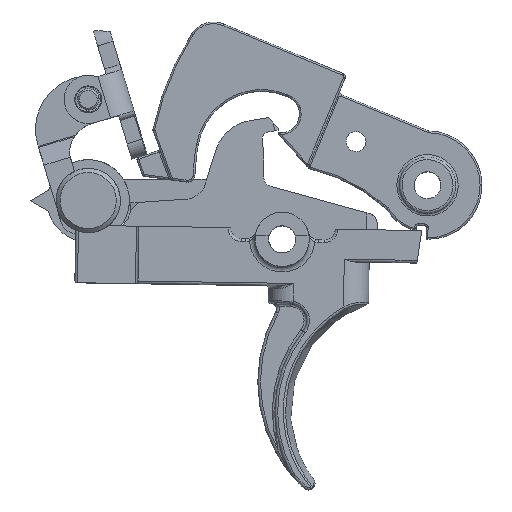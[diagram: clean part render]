
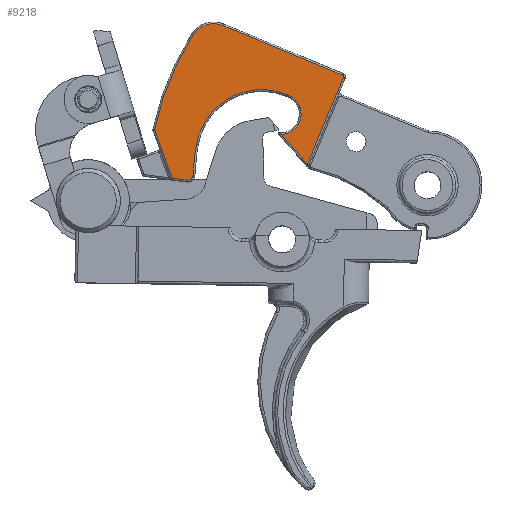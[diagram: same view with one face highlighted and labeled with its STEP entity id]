
A CAD part, top view. The second image highlights one B-rep face of the part: STEP entity #9218.
In plain terms, the highlighted planar face has unit normal (0, 0, 1).
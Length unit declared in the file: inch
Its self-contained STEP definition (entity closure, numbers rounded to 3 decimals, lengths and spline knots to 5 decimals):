
#1012=CIRCLE('',#10325,0.01);
#1057=CIRCLE('',#10414,0.031);
#1059=CIRCLE('',#10417,1.36056);
#1061=CIRCLE('',#10420,0.385);
#1063=CIRCLE('',#10424,0.11935);
#1076=CIRCLE('',#10447,0.141);
#1078=CIRCLE('',#10450,1.615);
#1248=PLANE('',#10457);
#1818=FACE_OUTER_BOUND('',#2459,.T.);
#2459=EDGE_LOOP('',(#8425,#8426,#8427,#8428,#8429,#8430,#8431,#8432,#8433,
#8434,#8435,#8436,#8437));
#2919=LINE('',#24606,#3483);
#2961=LINE('',#24880,#3525);
#3017=LINE('',#25762,#3581);
#3021=LINE('',#25791,#3585);
#3023=LINE('',#25796,#3587);
#3024=LINE('',#25798,#3588);
#3483=VECTOR('',#12593,0.3937);
#3525=VECTOR('',#12785,0.3937);
#3581=VECTOR('',#13173,0.3937);
#3585=VECTOR('',#13215,0.3937);
#3587=VECTOR('',#13221,0.3937);
#3588=VECTOR('',#13224,0.3937);
#4276=VERTEX_POINT('',#24519);
#4290=VERTEX_POINT('',#24604);
#4350=VERTEX_POINT('',#24866);
#4353=VERTEX_POINT('',#24878);
#4406=VERTEX_POINT('',#25387);
#4438=VERTEX_POINT('',#25682);
#4440=VERTEX_POINT('',#25748);
#4441=VERTEX_POINT('',#25752);
#4442=VERTEX_POINT('',#25756);
#4443=VERTEX_POINT('',#25760);
#4448=VERTEX_POINT('',#25782);
#4450=VERTEX_POINT('',#25794);
#4452=VERTEX_POINT('',#25802);
#5502=EDGE_CURVE('',#4290,#4276,#2919,.T.);
#5596=EDGE_CURVE('',#4353,#4350,#2961,.T.);
#5672=EDGE_CURVE('',#4406,#4290,#1012,.T.);
#5750=EDGE_CURVE('',#4440,#4353,#1057,.T.);
#5752=EDGE_CURVE('',#4441,#4440,#1059,.T.);
#5754=EDGE_CURVE('',#4442,#4441,#1061,.T.);
#5756=EDGE_CURVE('',#4443,#4442,#3017,.T.);
#5757=EDGE_CURVE('',#4438,#4443,#1063,.T.);
#5771=EDGE_CURVE('',#4350,#4448,#3021,.T.);
#5774=EDGE_CURVE('',#4450,#4406,#3023,.T.);
#5775=EDGE_CURVE('',#4276,#4438,#3024,.T.);
#5778=EDGE_CURVE('',#4452,#4450,#1076,.T.);
#5780=EDGE_CURVE('',#4448,#4452,#1078,.T.);
#8425=ORIENTED_EDGE('',*,*,#5771,.F.);
#8426=ORIENTED_EDGE('',*,*,#5596,.F.);
#8427=ORIENTED_EDGE('',*,*,#5750,.F.);
#8428=ORIENTED_EDGE('',*,*,#5752,.F.);
#8429=ORIENTED_EDGE('',*,*,#5754,.F.);
#8430=ORIENTED_EDGE('',*,*,#5756,.F.);
#8431=ORIENTED_EDGE('',*,*,#5757,.F.);
#8432=ORIENTED_EDGE('',*,*,#5775,.F.);
#8433=ORIENTED_EDGE('',*,*,#5502,.F.);
#8434=ORIENTED_EDGE('',*,*,#5672,.F.);
#8435=ORIENTED_EDGE('',*,*,#5774,.F.);
#8436=ORIENTED_EDGE('',*,*,#5778,.F.);
#8437=ORIENTED_EDGE('',*,*,#5780,.F.);
#9218=ADVANCED_FACE('',(#1818),#1248,.T.);
#10325=AXIS2_PLACEMENT_3D('',#25389,#12951,#12952);
#10414=AXIS2_PLACEMENT_3D('',#25750,#13155,#13156);
#10417=AXIS2_PLACEMENT_3D('',#25754,#13161,#13162);
#10420=AXIS2_PLACEMENT_3D('',#25758,#13167,#13168);
#10424=AXIS2_PLACEMENT_3D('',#25764,#13176,#13177);
#10447=AXIS2_PLACEMENT_3D('',#25804,#13230,#13231);
#10450=AXIS2_PLACEMENT_3D('',#25807,#13236,#13237);
#10457=AXIS2_PLACEMENT_3D('',#25816,#13252,#13253);
#12593=DIRECTION('',(-0.358,-0.934,0.));
#12785=DIRECTION('',(-0.995,0.105,0.));
#12951=DIRECTION('center_axis',(0.,0.,-1.));
#12952=DIRECTION('ref_axis',(0.914,0.407,0.));
#13155=DIRECTION('center_axis',(0.,0.,-1.));
#13156=DIRECTION('ref_axis',(0.663,-0.748,0.));
#13161=DIRECTION('center_axis',(0.,0.,1.));
#13162=DIRECTION('ref_axis',(-0.997,0.081,0.));
#13167=DIRECTION('center_axis',(0.,0.,1.));
#13168=DIRECTION('ref_axis',(-0.504,0.863,0.));
#13173=DIRECTION('',(-0.934,0.358,0.));
#13176=DIRECTION('center_axis',(0.,0.,1.));
#13177=DIRECTION('ref_axis',(0.979,-0.204,0.));
#13215=DIRECTION('',(-0.371,0.929,0.));
#13221=DIRECTION('',(0.934,-0.358,0.));
#13224=DIRECTION('',(-0.688,0.725,0.));
#13230=DIRECTION('center_axis',(0.,0.,-1.));
#13231=DIRECTION('ref_axis',(-0.325,0.946,0.));
#13236=DIRECTION('center_axis',(0.,0.,-1.));
#13237=DIRECTION('ref_axis',(-0.937,0.349,0.));
#13252=DIRECTION('center_axis',(0.,0.,1.));
#13253=DIRECTION('ref_axis',(1.,0.,0.));
#24519=CARTESIAN_POINT('',(-0.69934,0.10356,0.3));
#24604=CARTESIAN_POINT('',(-0.50441,0.61137,0.3));
#24606=CARTESIAN_POINT('',(-0.58907,0.39082,0.3));
#24866=CARTESIAN_POINT('',(-1.48028,-0.00027,0.3));
#24878=CARTESIAN_POINT('',(-1.39463,-0.00927,0.3));
#24880=CARTESIAN_POINT('',(-1.22169,-0.02745,0.3));
#25387=CARTESIAN_POINT('',(-0.51016,0.62429,0.3));
#25389=CARTESIAN_POINT('Origin',(-0.51374,0.61495,0.3));
#25682=CARTESIAN_POINT('',(-0.85704,0.26974,0.3));
#25748=CARTESIAN_POINT('',(-1.3604,0.02108,0.3));
#25750=CARTESIAN_POINT('Origin',(-1.39139,0.02156,0.3));
#25752=CARTESIAN_POINT('',(-1.34582,0.19973,0.3));
#25754=CARTESIAN_POINT('Origin',(0.,0.,0.3));
#25756=CARTESIAN_POINT('',(-0.827,0.50276,0.3));
#25758=CARTESIAN_POINT('Origin',(-0.96497,0.14334,0.3));
#25760=CARTESIAN_POINT('',(-0.8207,0.50034,0.3));
#25762=CARTESIAN_POINT('',(-0.76165,0.47768,0.3));
#25764=CARTESIAN_POINT('Origin',(-0.86347,0.38892,0.3));
#25782=CARTESIAN_POINT('',(-1.59102,0.27729,0.3));
#25791=CARTESIAN_POINT('',(-1.53857,0.14584,0.3));
#25794=CARTESIAN_POINT('',(-1.21134,0.89345,0.3));
#25796=CARTESIAN_POINT('',(-0.55322,0.64082,0.3));
#25798=CARTESIAN_POINT('',(-0.84495,0.25699,0.3));
#25802=CARTESIAN_POINT('',(-1.38258,0.83469,0.3));
#25804=CARTESIAN_POINT('Origin',(-1.26187,0.76181,0.3));
#25807=CARTESIAN_POINT('Origin',(0.,0.,0.3));
#25816=CARTESIAN_POINT('Origin',(-0.75349,0.30363,0.3));
